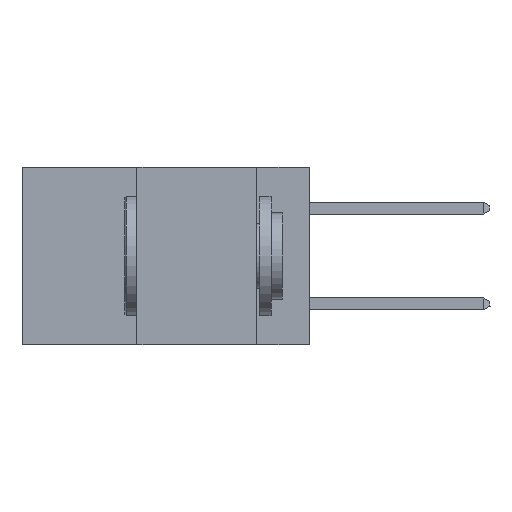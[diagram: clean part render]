
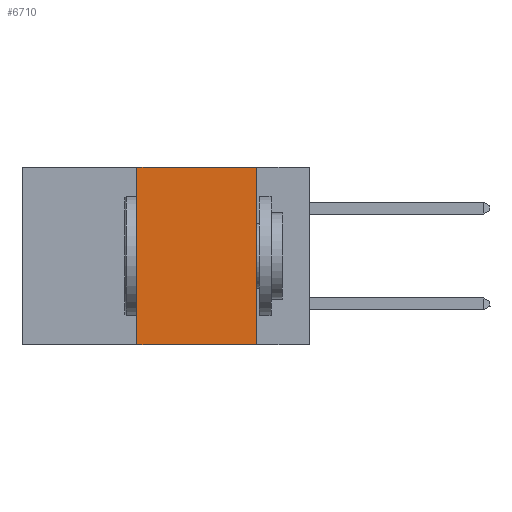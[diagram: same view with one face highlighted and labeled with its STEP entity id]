
A CAD part, left-side view. The second image highlights one B-rep face of the part: STEP entity #6710.
In plain terms, the highlighted planar face has unit normal (-1, 0, 0).
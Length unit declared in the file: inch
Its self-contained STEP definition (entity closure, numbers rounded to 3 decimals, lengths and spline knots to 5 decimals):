
#14 = CARTESIAN_POINT ( 'NONE',  ( 0., 0.36, 0. ) ) ;
#967 = VECTOR ( 'NONE', #8511, 39.37008 ) ;
#1706 = CARTESIAN_POINT ( 'NONE',  ( 0., 0.11, 0. ) ) ;
#1876 = EDGE_CURVE ( 'NONE', #19161, #12473, #11279, .T. ) ;
#3083 = EDGE_CURVE ( 'NONE', #19410, #7475, #6845, .T. ) ;
#4031 = ORIENTED_EDGE ( 'NONE', *, *, #4498, .T. ) ;
#4498 = EDGE_CURVE ( 'NONE', #19410, #12473, #20264, .T. ) ;
#5129 = CARTESIAN_POINT ( 'NONE',  ( 0., 0.6, -0.37 ) ) ;
#6710 = ADVANCED_FACE ( 'NONE', ( #9044 ), #16536, .F. ) ;
#6845 = LINE ( 'NONE', #14, #21092 ) ;
#7452 = CARTESIAN_POINT ( 'NONE',  ( 0., 0.36, 0. ) ) ;
#7475 = VERTEX_POINT ( 'NONE', #7452 ) ;
#7641 = ORIENTED_EDGE ( 'NONE', *, *, #3083, .F. ) ;
#8511 = DIRECTION ( 'NONE',  ( 0., 0., -1. ) ) ;
#8653 = AXIS2_PLACEMENT_3D ( 'NONE', #17897, #16327, #19663 ) ;
#9044 = FACE_OUTER_BOUND ( 'NONE', #12970, .T. ) ;
#9060 = EDGE_CURVE ( 'NONE', #7475, #19161, #18735, .T. ) ;
#9757 = DIRECTION ( 'NONE',  ( 0., 0., 1. ) ) ;
#9772 = CARTESIAN_POINT ( 'NONE',  ( 0., 0.36, -0.37 ) ) ;
#11279 = LINE ( 'NONE', #1706, #967 ) ;
#12473 = VERTEX_POINT ( 'NONE', #19953 ) ;
#12970 = EDGE_LOOP ( 'NONE', ( #19476, #18853, #7641, #4031 ) ) ;
#14442 = CARTESIAN_POINT ( 'NONE',  ( 0., 0.6, 0. ) ) ;
#16327 = DIRECTION ( 'NONE',  ( 1., 0., 0. ) ) ;
#16536 = PLANE ( 'NONE',  #8653 ) ;
#17897 = CARTESIAN_POINT ( 'NONE',  ( 0., 0.6, 0. ) ) ;
#18735 = LINE ( 'NONE', #14442, #20841 ) ;
#18853 = ORIENTED_EDGE ( 'NONE', *, *, #9060, .F. ) ;
#19148 = DIRECTION ( 'NONE',  ( 0., -1., 0. ) ) ;
#19161 = VERTEX_POINT ( 'NONE', #20865 ) ;
#19410 = VERTEX_POINT ( 'NONE', #9772 ) ;
#19476 = ORIENTED_EDGE ( 'NONE', *, *, #1876, .F. ) ;
#19663 = DIRECTION ( 'NONE',  ( 0., 0., -1. ) ) ;
#19753 = VECTOR ( 'NONE', #20085, 39.37008 ) ;
#19953 = CARTESIAN_POINT ( 'NONE',  ( 0., 0.11, -0.37 ) ) ;
#20085 = DIRECTION ( 'NONE',  ( 0., -1., 0. ) ) ;
#20264 = LINE ( 'NONE', #5129, #19753 ) ;
#20841 = VECTOR ( 'NONE', #19148, 39.37008 ) ;
#20865 = CARTESIAN_POINT ( 'NONE',  ( 0., 0.11, 0. ) ) ;
#21092 = VECTOR ( 'NONE', #9757, 39.37008 ) ;
